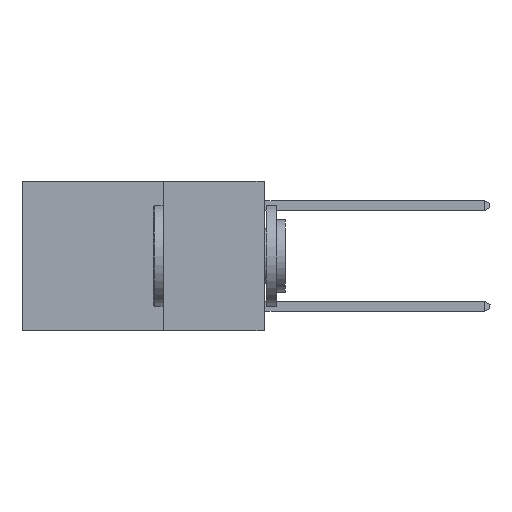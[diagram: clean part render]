
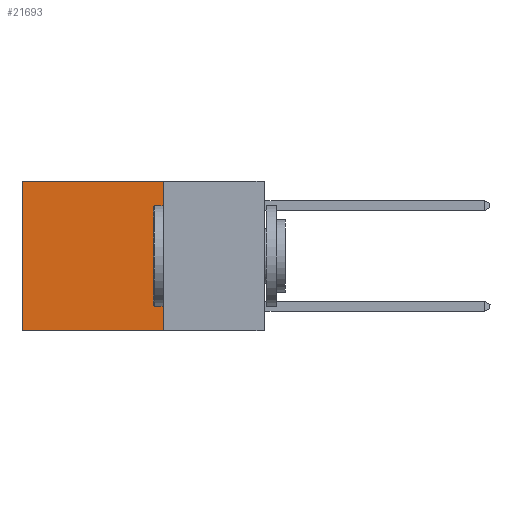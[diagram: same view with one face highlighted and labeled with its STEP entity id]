
A CAD part, left-side view. The second image highlights one B-rep face of the part: STEP entity #21693.
In plain terms, the highlighted planar face has unit normal (-1, 0, 0).
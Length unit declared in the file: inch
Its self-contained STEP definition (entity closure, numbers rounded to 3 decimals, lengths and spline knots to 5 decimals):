
#199 = LINE ( 'NONE', #12669, #17581 ) ;
#606 = EDGE_LOOP ( 'NONE', ( #12901, #22085, #16687, #14281 ) ) ;
#660 = VECTOR ( 'NONE', #8823, 39.37008 ) ;
#759 = LINE ( 'NONE', #7360, #14099 ) ;
#950 = VERTEX_POINT ( 'NONE', #16195 ) ;
#4113 = DIRECTION ( 'NONE',  ( 0., 1., 0. ) ) ;
#4131 = DIRECTION ( 'NONE',  ( 1., 0., 0. ) ) ;
#4508 = LINE ( 'NONE', #17193, #22150 ) ;
#5841 = VERTEX_POINT ( 'NONE', #12073 ) ;
#6915 = EDGE_CURVE ( 'NONE', #5841, #950, #4508, .T. ) ;
#7360 = CARTESIAN_POINT ( 'NONE',  ( 0.2625, 0.25, -0.37 ) ) ;
#7507 = PLANE ( 'NONE',  #20058 ) ;
#8662 = EDGE_CURVE ( 'NONE', #5841, #14892, #199, .T. ) ;
#8670 = DIRECTION ( 'NONE',  ( 0., 0., -1. ) ) ;
#8823 = DIRECTION ( 'NONE',  ( 0., 0., -1. ) ) ;
#9084 = DIRECTION ( 'NONE',  ( 0., 1., 0. ) ) ;
#9432 = LINE ( 'NONE', #19072, #660 ) ;
#10542 = VERTEX_POINT ( 'NONE', #13773 ) ;
#10957 = CARTESIAN_POINT ( 'NONE',  ( 0.2625, 0.25, 0. ) ) ;
#11485 = EDGE_CURVE ( 'NONE', #950, #10542, #759, .T. ) ;
#12073 = CARTESIAN_POINT ( 'NONE',  ( 0.2625, 0.25, 0. ) ) ;
#12669 = CARTESIAN_POINT ( 'NONE',  ( 0.2625, 0.25, 0. ) ) ;
#12901 = ORIENTED_EDGE ( 'NONE', *, *, #19079, .T. ) ;
#13773 = CARTESIAN_POINT ( 'NONE',  ( 0.2625, 0.6, -0.37 ) ) ;
#14099 = VECTOR ( 'NONE', #9084, 39.37008 ) ;
#14281 = ORIENTED_EDGE ( 'NONE', *, *, #8662, .T. ) ;
#14892 = VERTEX_POINT ( 'NONE', #19487 ) ;
#16103 = DIRECTION ( 'NONE',  ( 0., 0., -1. ) ) ;
#16195 = CARTESIAN_POINT ( 'NONE',  ( 0.2625, 0.25, -0.37 ) ) ;
#16687 = ORIENTED_EDGE ( 'NONE', *, *, #6915, .F. ) ;
#17193 = CARTESIAN_POINT ( 'NONE',  ( 0.2625, 0.25, 0. ) ) ;
#17581 = VECTOR ( 'NONE', #4113, 39.37008 ) ;
#19072 = CARTESIAN_POINT ( 'NONE',  ( 0.2625, 0.6, 0. ) ) ;
#19079 = EDGE_CURVE ( 'NONE', #14892, #10542, #9432, .T. ) ;
#19487 = CARTESIAN_POINT ( 'NONE',  ( 0.2625, 0.6, 0. ) ) ;
#20058 = AXIS2_PLACEMENT_3D ( 'NONE', #10957, #4131, #16103 ) ;
#21132 = FACE_OUTER_BOUND ( 'NONE', #606, .T. ) ;
#21693 = ADVANCED_FACE ( 'NONE', ( #21132 ), #7507, .F. ) ;
#22085 = ORIENTED_EDGE ( 'NONE', *, *, #11485, .F. ) ;
#22150 = VECTOR ( 'NONE', #8670, 39.37008 ) ;
